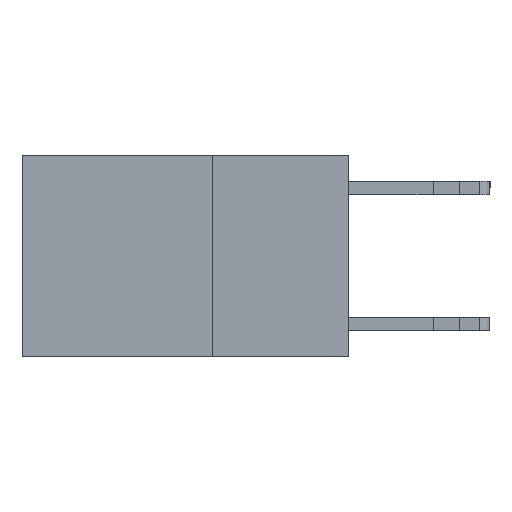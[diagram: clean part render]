
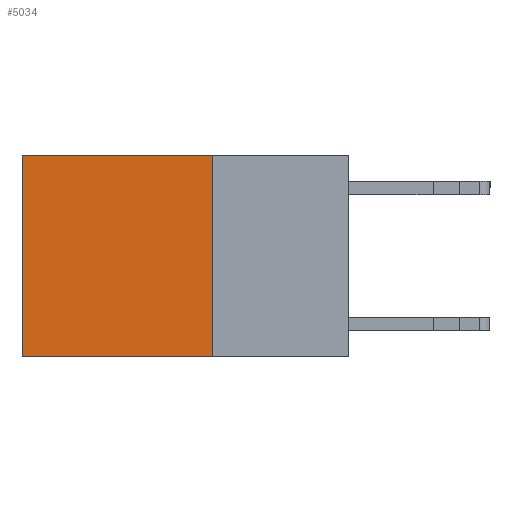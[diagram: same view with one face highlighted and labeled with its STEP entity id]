
A CAD part, left-side view. The second image highlights one B-rep face of the part: STEP entity #5034.
In plain terms, the highlighted planar face has unit normal (-1, 0, 0).
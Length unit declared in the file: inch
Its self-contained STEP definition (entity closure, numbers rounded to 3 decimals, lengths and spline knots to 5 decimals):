
#856 = VECTOR ( 'NONE', #5913, 39.37008 ) ;
#966 = CARTESIAN_POINT ( 'NONE',  ( 0.2625, 0.25, 0. ) ) ;
#1182 = ORIENTED_EDGE ( 'NONE', *, *, #14761, .T. ) ;
#1190 = FACE_OUTER_BOUND ( 'NONE', #2789, .T. ) ;
#2751 = CARTESIAN_POINT ( 'NONE',  ( 0.2625, 0.25, 0. ) ) ;
#2789 = EDGE_LOOP ( 'NONE', ( #1182, #12899, #10698, #8250 ) ) ;
#3348 = VECTOR ( 'NONE', #15125, 39.37008 ) ;
#3619 = PLANE ( 'NONE',  #7280 ) ;
#5034 = ADVANCED_FACE ( 'NONE', ( #1190 ), #3619, .F. ) ;
#5570 = LINE ( 'NONE', #9181, #3348 ) ;
#5913 = DIRECTION ( 'NONE',  ( 0., 1., 0. ) ) ;
#7166 = CARTESIAN_POINT ( 'NONE',  ( 0.2625, 0.25, 0. ) ) ;
#7280 = AXIS2_PLACEMENT_3D ( 'NONE', #966, #10516, #11893 ) ;
#7688 = VERTEX_POINT ( 'NONE', #9731 ) ;
#8250 = ORIENTED_EDGE ( 'NONE', *, *, #12170, .T. ) ;
#9088 = VERTEX_POINT ( 'NONE', #14108 ) ;
#9102 = LINE ( 'NONE', #9185, #11822 ) ;
#9142 = VECTOR ( 'NONE', #9840, 39.37008 ) ;
#9181 = CARTESIAN_POINT ( 'NONE',  ( 0.2625, 0.25, -0.37 ) ) ;
#9185 = CARTESIAN_POINT ( 'NONE',  ( 0.2625, 0.25, 0. ) ) ;
#9731 = CARTESIAN_POINT ( 'NONE',  ( 0.2625, 0.6, -0.37 ) ) ;
#9840 = DIRECTION ( 'NONE',  ( 0., 0., -1. ) ) ;
#10516 = DIRECTION ( 'NONE',  ( 1., 0., 0. ) ) ;
#10698 = ORIENTED_EDGE ( 'NONE', *, *, #12959, .F. ) ;
#11531 = EDGE_CURVE ( 'NONE', #13364, #7688, #5570, .T. ) ;
#11822 = VECTOR ( 'NONE', #13715, 39.37008 ) ;
#11841 = LINE ( 'NONE', #7166, #856 ) ;
#11893 = DIRECTION ( 'NONE',  ( 0., 0., -1. ) ) ;
#12170 = EDGE_CURVE ( 'NONE', #13494, #9088, #11841, .T. ) ;
#12708 = CARTESIAN_POINT ( 'NONE',  ( 0.2625, 0.25, -0.37 ) ) ;
#12899 = ORIENTED_EDGE ( 'NONE', *, *, #11531, .F. ) ;
#12959 = EDGE_CURVE ( 'NONE', #13494, #13364, #9102, .T. ) ;
#13342 = LINE ( 'NONE', #14904, #9142 ) ;
#13364 = VERTEX_POINT ( 'NONE', #12708 ) ;
#13494 = VERTEX_POINT ( 'NONE', #2751 ) ;
#13715 = DIRECTION ( 'NONE',  ( 0., 0., -1. ) ) ;
#14108 = CARTESIAN_POINT ( 'NONE',  ( 0.2625, 0.6, 0. ) ) ;
#14761 = EDGE_CURVE ( 'NONE', #9088, #7688, #13342, .T. ) ;
#14904 = CARTESIAN_POINT ( 'NONE',  ( 0.2625, 0.6, 0. ) ) ;
#15125 = DIRECTION ( 'NONE',  ( 0., 1., 0. ) ) ;
